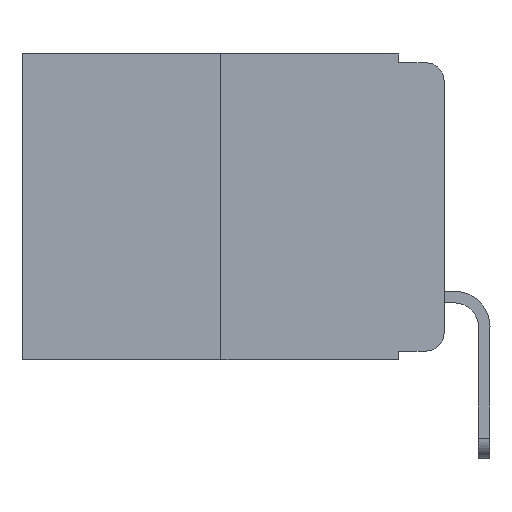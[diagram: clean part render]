
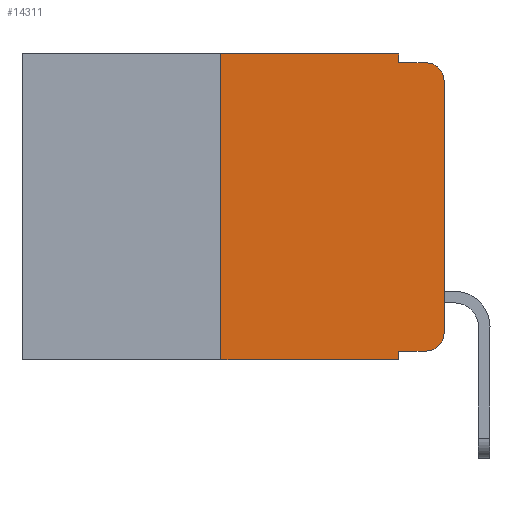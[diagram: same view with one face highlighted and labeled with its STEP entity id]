
A CAD part, left-side view. The second image highlights one B-rep face of the part: STEP entity #14311.
In plain terms, the highlighted planar face has unit normal (-1, 0, 0).
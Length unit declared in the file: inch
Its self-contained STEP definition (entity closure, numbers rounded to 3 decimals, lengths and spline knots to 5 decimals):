
#1062 = ORIENTED_EDGE ( 'NONE', *, *, #6822, .F. ) ;
#1164 = LINE ( 'NONE', #18180, #20628 ) ;
#1432 = VECTOR ( 'NONE', #21546, 39.37008 ) ;
#1594 = EDGE_CURVE ( 'NONE', #21928, #2220, #5190, .T. ) ;
#1819 = DIRECTION ( 'NONE',  ( -1., 0., 0. ) ) ;
#2220 = VERTEX_POINT ( 'NONE', #3361 ) ;
#2227 = LINE ( 'NONE', #11262, #20261 ) ;
#2824 = CIRCLE ( 'NONE', #13611, 0.02 ) ;
#3286 = CARTESIAN_POINT ( 'NONE',  ( 0., 0.051, -0.01 ) ) ;
#3361 = CARTESIAN_POINT ( 'NONE',  ( 0., 0.02, -0.01 ) ) ;
#3663 = VECTOR ( 'NONE', #8022, 39.37008 ) ;
#3948 = DIRECTION ( 'NONE',  ( -1., 0., 0. ) ) ;
#4192 = CARTESIAN_POINT ( 'NONE',  ( 0., 0.051, 0. ) ) ;
#4397 = ORIENTED_EDGE ( 'NONE', *, *, #7998, .F. ) ;
#4475 = ORIENTED_EDGE ( 'NONE', *, *, #10241, .T. ) ;
#4942 = CIRCLE ( 'NONE', #22187, 0.02 ) ;
#5190 = LINE ( 'NONE', #20011, #9669 ) ;
#5327 = VECTOR ( 'NONE', #11238, 39.37008 ) ;
#5332 = CARTESIAN_POINT ( 'NONE',  ( 0., 0.051, -0.333 ) ) ;
#5645 = VERTEX_POINT ( 'NONE', #9625 ) ;
#5846 = VERTEX_POINT ( 'NONE', #17582 ) ;
#6086 = EDGE_CURVE ( 'NONE', #5645, #6914, #1164, .T. ) ;
#6697 = CARTESIAN_POINT ( 'NONE',  ( 0., 0.051, -0.343 ) ) ;
#6775 = VERTEX_POINT ( 'NONE', #22398 ) ;
#6822 = EDGE_CURVE ( 'NONE', #14427, #21928, #8224, .T. ) ;
#6914 = VERTEX_POINT ( 'NONE', #8210 ) ;
#7273 = CARTESIAN_POINT ( 'NONE',  ( 0., 0.051, 0. ) ) ;
#7560 = DIRECTION ( 'NONE',  ( 0., -1., 0. ) ) ;
#7725 = CARTESIAN_POINT ( 'NONE',  ( 0., 0.473, -0.343 ) ) ;
#7927 = ORIENTED_EDGE ( 'NONE', *, *, #22760, .F. ) ;
#7998 = EDGE_CURVE ( 'NONE', #6914, #14427, #2227, .T. ) ;
#8022 = DIRECTION ( 'NONE',  ( 0., 0., 1. ) ) ;
#8210 = CARTESIAN_POINT ( 'NONE',  ( 0., 0.25, 0. ) ) ;
#8224 = LINE ( 'NONE', #4192, #11844 ) ;
#8668 = EDGE_CURVE ( 'NONE', #5645, #23028, #21927, .T. ) ;
#9147 = CARTESIAN_POINT ( 'NONE',  ( 0., 0., 0. ) ) ;
#9450 = ORIENTED_EDGE ( 'NONE', *, *, #18680, .T. ) ;
#9625 = CARTESIAN_POINT ( 'NONE',  ( 0., 0.25, -0.343 ) ) ;
#9658 = DIRECTION ( 'NONE',  ( 0., 0., -1. ) ) ;
#9669 = VECTOR ( 'NONE', #7560, 39.37008 ) ;
#9948 = PLANE ( 'NONE',  #14433 ) ;
#10241 = EDGE_CURVE ( 'NONE', #6775, #2220, #2824, .T. ) ;
#11122 = ORIENTED_EDGE ( 'NONE', *, *, #1594, .F. ) ;
#11238 = DIRECTION ( 'NONE',  ( 0., -1., 0. ) ) ;
#11262 = CARTESIAN_POINT ( 'NONE',  ( 0., 0.473, 0. ) ) ;
#11319 = CARTESIAN_POINT ( 'NONE',  ( 0., 0., -0.313 ) ) ;
#11844 = VECTOR ( 'NONE', #13358, 39.37008 ) ;
#12060 = LINE ( 'NONE', #9147, #3663 ) ;
#12567 = CARTESIAN_POINT ( 'NONE',  ( 0., 0.02, -0.03 ) ) ;
#13234 = ORIENTED_EDGE ( 'NONE', *, *, #19366, .T. ) ;
#13358 = DIRECTION ( 'NONE',  ( 0., 0., -1. ) ) ;
#13365 = EDGE_CURVE ( 'NONE', #5846, #14621, #4942, .T. ) ;
#13605 = VERTEX_POINT ( 'NONE', #20538 ) ;
#13611 = AXIS2_PLACEMENT_3D ( 'NONE', #12567, #3948, #21671 ) ;
#14311 = ADVANCED_FACE ( 'NONE', ( #19559 ), #9948, .F. ) ;
#14427 = VERTEX_POINT ( 'NONE', #7273 ) ;
#14433 = AXIS2_PLACEMENT_3D ( 'NONE', #18945, #21463, #23057 ) ;
#14621 = VERTEX_POINT ( 'NONE', #11319 ) ;
#14723 = ORIENTED_EDGE ( 'NONE', *, *, #13365, .T. ) ;
#15489 = EDGE_LOOP ( 'NONE', ( #13234, #4475, #11122, #1062, #4397, #18712, #20611, #7927, #9450, #14723 ) ) ;
#16559 = LINE ( 'NONE', #18005, #17976 ) ;
#17582 = CARTESIAN_POINT ( 'NONE',  ( 0., 0.02, -0.333 ) ) ;
#17784 = DIRECTION ( 'NONE',  ( 0., 0., -1. ) ) ;
#17976 = VECTOR ( 'NONE', #9658, 39.37008 ) ;
#18005 = CARTESIAN_POINT ( 'NONE',  ( 0., 0.051, 0. ) ) ;
#18180 = CARTESIAN_POINT ( 'NONE',  ( 0., 0.25, 0. ) ) ;
#18543 = DIRECTION ( 'NONE',  ( 0., -1., 0. ) ) ;
#18594 = LINE ( 'NONE', #5332, #1432 ) ;
#18680 = EDGE_CURVE ( 'NONE', #13605, #5846, #18594, .T. ) ;
#18712 = ORIENTED_EDGE ( 'NONE', *, *, #6086, .F. ) ;
#18945 = CARTESIAN_POINT ( 'NONE',  ( 0., 0.473, 0. ) ) ;
#19366 = EDGE_CURVE ( 'NONE', #14621, #6775, #12060, .T. ) ;
#19559 = FACE_OUTER_BOUND ( 'NONE', #15489, .T. ) ;
#20011 = CARTESIAN_POINT ( 'NONE',  ( 0., 0.051, -0.01 ) ) ;
#20261 = VECTOR ( 'NONE', #18543, 39.37008 ) ;
#20538 = CARTESIAN_POINT ( 'NONE',  ( 0., 0.051, -0.333 ) ) ;
#20611 = ORIENTED_EDGE ( 'NONE', *, *, #8668, .T. ) ;
#20628 = VECTOR ( 'NONE', #21907, 39.37008 ) ;
#21463 = DIRECTION ( 'NONE',  ( 1., 0., 0. ) ) ;
#21546 = DIRECTION ( 'NONE',  ( 0., -1., 0. ) ) ;
#21589 = CARTESIAN_POINT ( 'NONE',  ( 0., 0.02, -0.313 ) ) ;
#21671 = DIRECTION ( 'NONE',  ( 0., 0., -1. ) ) ;
#21907 = DIRECTION ( 'NONE',  ( 0., 0., 1. ) ) ;
#21927 = LINE ( 'NONE', #7725, #5327 ) ;
#21928 = VERTEX_POINT ( 'NONE', #3286 ) ;
#22187 = AXIS2_PLACEMENT_3D ( 'NONE', #21589, #1819, #17784 ) ;
#22398 = CARTESIAN_POINT ( 'NONE',  ( 0., 0., -0.03 ) ) ;
#22760 = EDGE_CURVE ( 'NONE', #13605, #23028, #16559, .T. ) ;
#23028 = VERTEX_POINT ( 'NONE', #6697 ) ;
#23057 = DIRECTION ( 'NONE',  ( 0., 0., -1. ) ) ;
